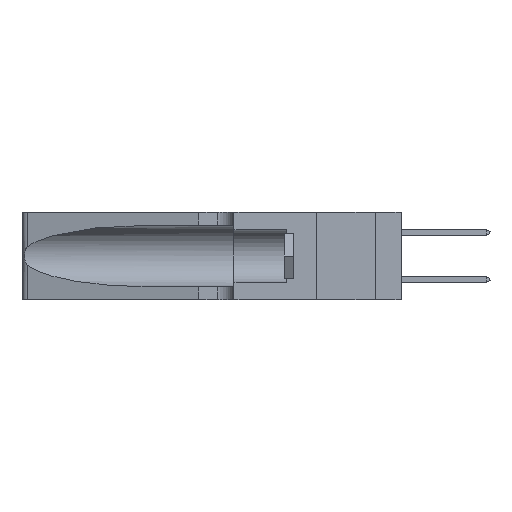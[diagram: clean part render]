
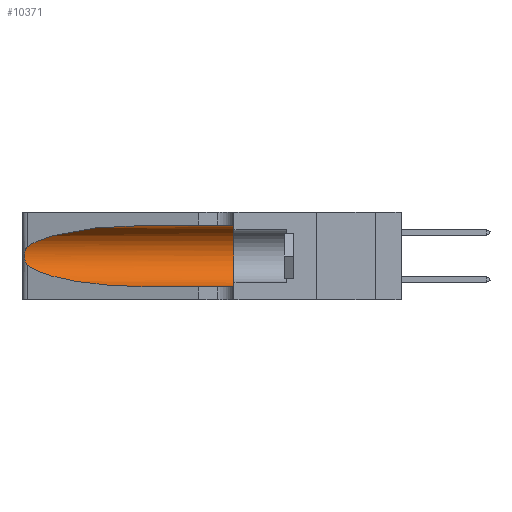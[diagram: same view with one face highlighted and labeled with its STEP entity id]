
A CAD part, left-side view. The second image highlights one B-rep face of the part: STEP entity #10371.
In plain terms, the highlighted cylindrical face has radius 3.308 mm (diameter 6.617 mm), a partial arc.
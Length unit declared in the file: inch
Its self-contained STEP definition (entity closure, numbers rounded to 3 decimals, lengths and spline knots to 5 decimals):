
#564 = CARTESIAN_POINT ( 'NONE',  ( 0.1305, 0.72297, 0.05475 ) ) ;
#622 = EDGE_CURVE ( 'NONE', #3451, #1385, #13762, .T. ) ;
#981 = AXIS2_PLACEMENT_3D ( 'NONE', #11087, #25111, #20878 ) ;
#1256 = CARTESIAN_POINT ( 'NONE',  ( 0.26075, 1.23896, 0.178 ) ) ;
#1385 = VERTEX_POINT ( 'NONE', #16842 ) ;
#2465 = CARTESIAN_POINT ( 'NONE',  ( 0.25487, 1.22718, 0.22369 ) ) ;
#2995 = CARTESIAN_POINT ( 'NONE',  ( 0.25639, 1.23186, 0.15144 ) ) ;
#3173 = CARTESIAN_POINT ( 'NONE',  ( 0.1305, 0.72297, 0.31525 ) ) ;
#3451 = VERTEX_POINT ( 'NONE', #3173 ) ;
#3891 = ORIENTED_EDGE ( 'NONE', *, *, #6601, .T. ) ;
#3954 = CARTESIAN_POINT ( 'NONE',  ( 0.25487, 1.22718, 0.14631 ) ) ;
#4306 = ORIENTED_EDGE ( 'NONE', *, *, #14980, .T. ) ;
#5247 = CARTESIAN_POINT ( 'NONE',  ( 0.1305, 0.72297, 0.31525 ) ) ;
#5330 = CARTESIAN_POINT ( 'NONE',  ( 0.2373, 1.15595, 0.28018 ) ) ;
#5605 = CARTESIAN_POINT ( 'NONE',  ( 0.1305, 0.35, 0.185 ) ) ;
#5801 = DIRECTION ( 'NONE',  ( 0., -1., 0. ) ) ;
#6601 = EDGE_CURVE ( 'NONE', #3451, #21768, #15171, .T. ) ;
#7012 = VERTEX_POINT ( 'NONE', #17133 ) ;
#8016 = ORIENTED_EDGE ( 'NONE', *, *, #19504, .F. ) ;
#8378 = EDGE_LOOP ( 'NONE', ( #3891, #20222, #21788, #4306, #8016, #9366 ) ) ;
#8971 = VERTEX_POINT ( 'NONE', #3954 ) ;
#9023 = CARTESIAN_POINT ( 'NONE',  ( 0.25789, 1.23486, 0.15765 ) ) ;
#9304 = CIRCLE ( 'NONE', #14312, 0.13025 ) ;
#9366 = ORIENTED_EDGE ( 'NONE', *, *, #622, .F. ) ;
#10371 = ADVANCED_FACE ( 'NONE', ( #25459 ), #24498, .F. ) ;
#11087 = CARTESIAN_POINT ( 'NONE',  ( 0.1305, 1.61858, 0.185 ) ) ;
#11191 = CARTESIAN_POINT ( 'NONE',  ( 0.25854, 1.2359, 0.20912 ) ) ;
#12547 = CARTESIAN_POINT ( 'NONE',  ( 0.25487, 1.22718, 0.14631 ) ) ;
#12575 = VECTOR ( 'NONE', #17236, 39.37008 ) ;
#12629 = VERTEX_POINT ( 'NONE', #15896 ) ;
#12905 = CARTESIAN_POINT ( 'NONE',  ( 0.26018, 1.23835, 0.19895 ) ) ;
#12984 = CARTESIAN_POINT ( 'NONE',  ( 0.26017, 1.23833, 0.17102 ) ) ;
#13762 = LINE ( 'NONE', #17452, #14333 ) ;
#14312 = AXIS2_PLACEMENT_3D ( 'NONE', #5605, #19315, #25265 ) ;
#14333 = VECTOR ( 'NONE', #5801, 39.37008 ) ;
#14519 = CARTESIAN_POINT ( 'NONE',  ( 0.2373, 1.15595, 0.08982 ) ) ;
#14877 = CARTESIAN_POINT ( 'NONE',  ( 0.25639, 1.23184, 0.21858 ) ) ;
#14960 = CARTESIAN_POINT ( 'NONE',  ( 0.25487, 1.22718, 0.22369 ) ) ;
#14980 = EDGE_CURVE ( 'NONE', #12629, #7012, #20892, .T. ) ;
#15032 = CARTESIAN_POINT ( 'NONE',  ( 0.25787, 1.23484, 0.2124 ) ) ;
#15121 = CARTESIAN_POINT ( 'NONE',  ( 0.26075, 1.23896, 0.19203 ) ) ;
#15171 =( BOUNDED_CURVE ( )  B_SPLINE_CURVE ( 3, ( #5247, #17118, #5330, #25072 ),
 .UNSPECIFIED., .F., .F. ) 
 B_SPLINE_CURVE_WITH_KNOTS ( ( 4, 4 ),
 ( 1.5708, 2.84003 ),
 .UNSPECIFIED. ) 
 CURVE ( )  GEOMETRIC_REPRESENTATION_ITEM ( )  RATIONAL_B_SPLINE_CURVE ( ( 1., 0.87, 0.87, 1. ) ) 
 REPRESENTATION_ITEM ( '' )  );
#15896 = CARTESIAN_POINT ( 'NONE',  ( 0.1305, 0.72297, 0.05475 ) ) ;
#16663 = CARTESIAN_POINT ( 'NONE',  ( 0.18966, 0.96281, 0.05475 ) ) ;
#16777 = EDGE_CURVE ( 'NONE', #21768, #8971, #20994, .T. ) ;
#16833 = CARTESIAN_POINT ( 'NONE',  ( 0.25487, 1.22718, 0.14631 ) ) ;
#16842 = CARTESIAN_POINT ( 'NONE',  ( 0.1305, 0.35, 0.31525 ) ) ;
#16996 = CARTESIAN_POINT ( 'NONE',  ( 0.25555, 1.22994, 0.2215 ) ) ;
#17118 = CARTESIAN_POINT ( 'NONE',  ( 0.18966, 0.96281, 0.31525 ) ) ;
#17133 = CARTESIAN_POINT ( 'NONE',  ( 0.1305, 0.35, 0.05475 ) ) ;
#17140 = CARTESIAN_POINT ( 'NONE',  ( 0.1305, 1.61858, 0.05475 ) ) ;
#17236 = DIRECTION ( 'NONE',  ( 0., -1., 0. ) ) ;
#17452 = CARTESIAN_POINT ( 'NONE',  ( 0.1305, 1.61858, 0.31525 ) ) ;
#17853 =( BOUNDED_CURVE ( )  B_SPLINE_CURVE ( 3, ( #12547, #14519, #16663, #564 ),
 .UNSPECIFIED., .F., .T. ) 
 B_SPLINE_CURVE_WITH_KNOTS ( ( 4, 4 ),
 ( 3.44316, 4.71239 ),
 .UNSPECIFIED. ) 
 CURVE ( )  GEOMETRIC_REPRESENTATION_ITEM ( )  RATIONAL_B_SPLINE_CURVE ( ( 1., 0.87, 0.87, 1. ) ) 
 REPRESENTATION_ITEM ( '' )  );
#18937 = CARTESIAN_POINT ( 'NONE',  ( 0.25555, 1.22993, 0.14849 ) ) ;
#19315 = DIRECTION ( 'NONE',  ( 0., 1., 0. ) ) ;
#19504 = EDGE_CURVE ( 'NONE', #1385, #7012, #9304, .T. ) ;
#20222 = ORIENTED_EDGE ( 'NONE', *, *, #16777, .T. ) ;
#20643 = CARTESIAN_POINT ( 'NONE',  ( 0.25856, 1.23593, 0.16098 ) ) ;
#20878 = DIRECTION ( 'NONE',  ( 0., 0., -1. ) ) ;
#20892 = LINE ( 'NONE', #17140, #12575 ) ;
#20994 = B_SPLINE_CURVE_WITH_KNOTS ( 'NONE', 3,
 ( #14960, #16996, #14877, #15032, #11191, #12905, #15121, #1256, #12984, #20643, #9023, #2995, #18937, #16833 ),
 .UNSPECIFIED., .F., .F.,
 ( 4, 2, 2, 2, 2, 2, 4 ),
 ( 0., 0.00027, 0.00053, 0.00107, 0.0016, 0.00187, 0.00214 ),
 .UNSPECIFIED. ) ;
#21768 = VERTEX_POINT ( 'NONE', #2465 ) ;
#21788 = ORIENTED_EDGE ( 'NONE', *, *, #23620, .T. ) ;
#23620 = EDGE_CURVE ( 'NONE', #8971, #12629, #17853, .T. ) ;
#24498 = CYLINDRICAL_SURFACE ( 'NONE', #981, 0.13025 ) ;
#25072 = CARTESIAN_POINT ( 'NONE',  ( 0.25487, 1.22718, 0.22369 ) ) ;
#25111 = DIRECTION ( 'NONE',  ( 0., -1., 0. ) ) ;
#25265 = DIRECTION ( 'NONE',  ( 0., 0., 1. ) ) ;
#25459 = FACE_OUTER_BOUND ( 'NONE', #8378, .T. ) ;
